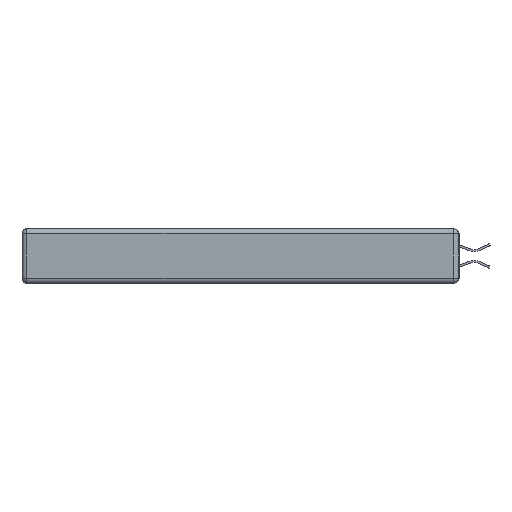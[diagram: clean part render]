
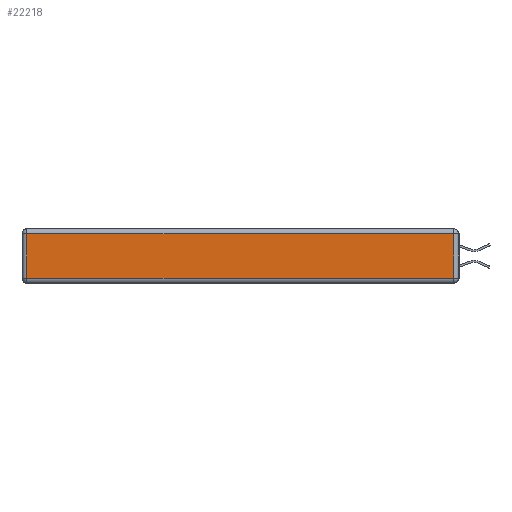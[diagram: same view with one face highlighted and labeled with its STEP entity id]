
A CAD part, left-side view. The second image highlights one B-rep face of the part: STEP entity #22218.
In plain terms, the highlighted planar face has unit normal (-1, 0, 0).
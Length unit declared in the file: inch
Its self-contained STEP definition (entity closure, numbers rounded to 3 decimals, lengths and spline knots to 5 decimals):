
#743 = CARTESIAN_POINT ( 'NONE',  ( 0., 0.03, -0.313 ) ) ;
#826 = VECTOR ( 'NONE', #10908, 39.37008 ) ;
#1459 = DIRECTION ( 'NONE',  ( 0., 0., 1. ) ) ;
#2290 = CARTESIAN_POINT ( 'NONE',  ( 0., 0.03, -0.03 ) ) ;
#2619 = LINE ( 'NONE', #5554, #826 ) ;
#2751 = DIRECTION ( 'NONE',  ( -1., 0., 0. ) ) ;
#3127 = VECTOR ( 'NONE', #14919, 39.37008 ) ;
#4534 = CARTESIAN_POINT ( 'NONE',  ( 0., 2.72, -0.313 ) ) ;
#5337 = AXIS2_PLACEMENT_3D ( 'NONE', #12152, #2751, #23390 ) ;
#5554 = CARTESIAN_POINT ( 'NONE',  ( 0., 0., -0.313 ) ) ;
#6104 = LINE ( 'NONE', #20712, #3127 ) ;
#6373 = EDGE_CURVE ( 'NONE', #12054, #8877, #6104, .T. ) ;
#8877 = VERTEX_POINT ( 'NONE', #4534 ) ;
#9047 = CARTESIAN_POINT ( 'NONE',  ( 0., 0.03, -0.343 ) ) ;
#9324 = VECTOR ( 'NONE', #1459, 39.37008 ) ;
#9535 = EDGE_CURVE ( 'NONE', #8877, #17689, #2619, .T. ) ;
#10603 = ORIENTED_EDGE ( 'NONE', *, *, #6373, .T. ) ;
#10714 = EDGE_LOOP ( 'NONE', ( #21844, #14338, #18846, #10603 ) ) ;
#10908 = DIRECTION ( 'NONE',  ( 0., -1., 0. ) ) ;
#12054 = VERTEX_POINT ( 'NONE', #12712 ) ;
#12080 = PLANE ( 'NONE',  #5337 ) ;
#12152 = CARTESIAN_POINT ( 'NONE',  ( 0., 0., -0.343 ) ) ;
#12712 = CARTESIAN_POINT ( 'NONE',  ( 0., 2.72, -0.03 ) ) ;
#14310 = VECTOR ( 'NONE', #23498, 39.37008 ) ;
#14338 = ORIENTED_EDGE ( 'NONE', *, *, #16390, .T. ) ;
#14919 = DIRECTION ( 'NONE',  ( 0., 0., -1. ) ) ;
#16390 = EDGE_CURVE ( 'NONE', #17689, #18541, #21418, .T. ) ;
#16834 = EDGE_CURVE ( 'NONE', #18541, #12054, #17550, .T. ) ;
#17460 = FACE_OUTER_BOUND ( 'NONE', #10714, .T. ) ;
#17483 = CARTESIAN_POINT ( 'NONE',  ( 0., 2.75, -0.03 ) ) ;
#17550 = LINE ( 'NONE', #17483, #14310 ) ;
#17689 = VERTEX_POINT ( 'NONE', #743 ) ;
#18541 = VERTEX_POINT ( 'NONE', #2290 ) ;
#18846 = ORIENTED_EDGE ( 'NONE', *, *, #16834, .T. ) ;
#20712 = CARTESIAN_POINT ( 'NONE',  ( 0., 2.72, -0.343 ) ) ;
#21418 = LINE ( 'NONE', #9047, #9324 ) ;
#21844 = ORIENTED_EDGE ( 'NONE', *, *, #9535, .T. ) ;
#22218 = ADVANCED_FACE ( 'NONE', ( #17460 ), #12080, .T. ) ;
#23390 = DIRECTION ( 'NONE',  ( 0., 0., 1. ) ) ;
#23498 = DIRECTION ( 'NONE',  ( 0., 1., 0. ) ) ;
